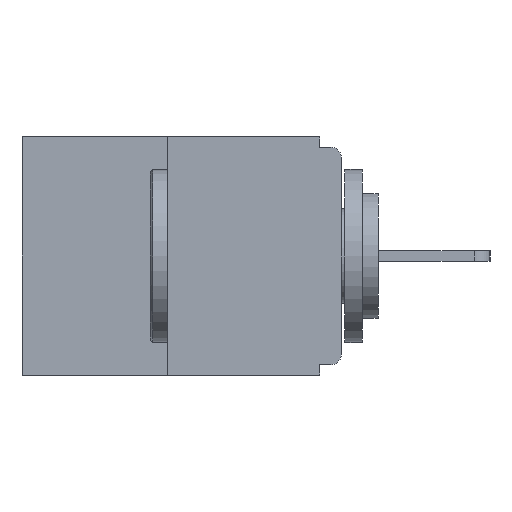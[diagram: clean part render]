
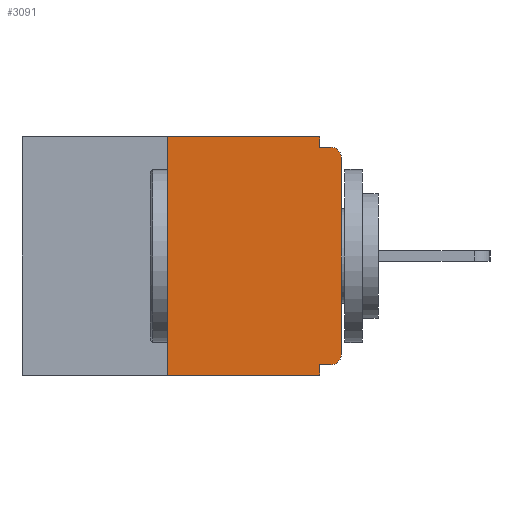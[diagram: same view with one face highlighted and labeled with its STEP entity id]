
A CAD part, left-side view. The second image highlights one B-rep face of the part: STEP entity #3091.
In plain terms, the highlighted planar face has unit normal (-1, 0, 0).
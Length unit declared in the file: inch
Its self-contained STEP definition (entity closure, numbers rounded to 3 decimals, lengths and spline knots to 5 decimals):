
#106 = EDGE_CURVE ( 'NONE', #6109, #9605, #8327, .T. ) ;
#162 = EDGE_CURVE ( 'NONE', #6109, #3119, #6458, .T. ) ;
#165 = EDGE_CURVE ( 'NONE', #1529, #3119, #3879, .T. ) ;
#190 = EDGE_CURVE ( 'NONE', #12623, #11741, #5471, .T. ) ;
#528 = CARTESIAN_POINT ( 'NONE',  ( 0., 0.015, -0.03 ) ) ;
#789 = EDGE_LOOP ( 'NONE', ( #4672, #4776, #4909, #4912, #4935, #4993, #5060, #5098, #5124, #5226 ) ) ;
#1015 = CARTESIAN_POINT ( 'NONE',  ( 0., 0.031, 0. ) ) ;
#1192 = CARTESIAN_POINT ( 'NONE',  ( 0., 0.46, 0. ) ) ;
#1377 = DIRECTION ( 'NONE',  ( 0., 0., 1. ) ) ;
#1440 = DIRECTION ( 'NONE',  ( 0., 1., 0. ) ) ;
#1529 = VERTEX_POINT ( 'NONE', #3378 ) ;
#1629 = VERTEX_POINT ( 'NONE', #12802 ) ;
#1872 = DIRECTION ( 'NONE',  ( 0., 0., -1. ) ) ;
#2788 = CARTESIAN_POINT ( 'NONE',  ( 0., 0.25, 0. ) ) ;
#2852 = LINE ( 'NONE', #1192, #8213 ) ;
#3022 = VERTEX_POINT ( 'NONE', #9345 ) ;
#3091 = ADVANCED_FACE ( 'NONE', ( #6620 ), #8493, .F. ) ;
#3107 = CARTESIAN_POINT ( 'NONE',  ( 0., 0.015, -0.328 ) ) ;
#3119 = VERTEX_POINT ( 'NONE', #13048 ) ;
#3264 = CARTESIAN_POINT ( 'NONE',  ( 0., 0., -0.015 ) ) ;
#3326 = CARTESIAN_POINT ( 'NONE',  ( 0., 0.031, 0. ) ) ;
#3341 = CARTESIAN_POINT ( 'NONE',  ( 0., 0.25, 0. ) ) ;
#3378 = CARTESIAN_POINT ( 'NONE',  ( 0., 0.031, -0.328 ) ) ;
#3797 = CARTESIAN_POINT ( 'NONE',  ( 0., 0.015, -0.313 ) ) ;
#3879 = LINE ( 'NONE', #6142, #11432 ) ;
#4030 = AXIS2_PLACEMENT_3D ( 'NONE', #8640, #5219, #6201 ) ;
#4672 = ORIENTED_EDGE ( 'NONE', *, *, #8890, .F. ) ;
#4776 = ORIENTED_EDGE ( 'NONE', *, *, #106, .F. ) ;
#4909 = ORIENTED_EDGE ( 'NONE', *, *, #162, .T. ) ;
#4912 = ORIENTED_EDGE ( 'NONE', *, *, #165, .F. ) ;
#4935 = ORIENTED_EDGE ( 'NONE', *, *, #6349, .F. ) ;
#4943 = DIRECTION ( 'NONE',  ( 0., 0., -1. ) ) ;
#4993 = ORIENTED_EDGE ( 'NONE', *, *, #7695, .T. ) ;
#5060 = ORIENTED_EDGE ( 'NONE', *, *, #6079, .T. ) ;
#5098 = ORIENTED_EDGE ( 'NONE', *, *, #8484, .T. ) ;
#5124 = ORIENTED_EDGE ( 'NONE', *, *, #7417, .F. ) ;
#5219 = DIRECTION ( 'NONE',  ( 1., 0., 0. ) ) ;
#5226 = ORIENTED_EDGE ( 'NONE', *, *, #190, .F. ) ;
#5432 = CARTESIAN_POINT ( 'NONE',  ( 0., 0.46, -0.343 ) ) ;
#5471 = LINE ( 'NONE', #3326, #13027 ) ;
#5819 = VERTEX_POINT ( 'NONE', #3107 ) ;
#5946 = LINE ( 'NONE', #9600, #10651 ) ;
#5986 = VECTOR ( 'NONE', #1377, 39.37008 ) ;
#6079 = EDGE_CURVE ( 'NONE', #6556, #3022, #5946, .T. ) ;
#6109 = VERTEX_POINT ( 'NONE', #9650 ) ;
#6142 = CARTESIAN_POINT ( 'NONE',  ( 0., 0.031, -0.343 ) ) ;
#6144 = DIRECTION ( 'NONE',  ( 0., 0., -1. ) ) ;
#6201 = DIRECTION ( 'NONE',  ( 0., 0., -1. ) ) ;
#6349 = EDGE_CURVE ( 'NONE', #5819, #1529, #7826, .T. ) ;
#6458 = LINE ( 'NONE', #5432, #9108 ) ;
#6556 = VERTEX_POINT ( 'NONE', #7315 ) ;
#6620 = FACE_OUTER_BOUND ( 'NONE', #789, .T. ) ;
#6659 = DIRECTION ( 'NONE',  ( 0., 0., 1. ) ) ;
#7137 = DIRECTION ( 'NONE',  ( 0., 0., -1. ) ) ;
#7315 = CARTESIAN_POINT ( 'NONE',  ( 0., 0., -0.313 ) ) ;
#7417 = EDGE_CURVE ( 'NONE', #11741, #1629, #11213, .T. ) ;
#7695 = EDGE_CURVE ( 'NONE', #5819, #6556, #7800, .T. ) ;
#7800 = CIRCLE ( 'NONE', #13311, 0.015 ) ;
#7826 = LINE ( 'NONE', #8999, #8132 ) ;
#8132 = VECTOR ( 'NONE', #1440, 39.37008 ) ;
#8213 = VECTOR ( 'NONE', #11827, 39.37008 ) ;
#8219 = AXIS2_PLACEMENT_3D ( 'NONE', #528, #8337, #1872 ) ;
#8327 = LINE ( 'NONE', #2788, #5986 ) ;
#8337 = DIRECTION ( 'NONE',  ( -1., 0., 0. ) ) ;
#8484 = EDGE_CURVE ( 'NONE', #3022, #1629, #12208, .T. ) ;
#8493 = PLANE ( 'NONE',  #4030 ) ;
#8640 = CARTESIAN_POINT ( 'NONE',  ( 0., 0.46, 0. ) ) ;
#8890 = EDGE_CURVE ( 'NONE', #9605, #12623, #2852, .T. ) ;
#8999 = CARTESIAN_POINT ( 'NONE',  ( 0., 0., -0.328 ) ) ;
#9108 = VECTOR ( 'NONE', #10791, 39.37008 ) ;
#9345 = CARTESIAN_POINT ( 'NONE',  ( 0., 0., -0.03 ) ) ;
#9600 = CARTESIAN_POINT ( 'NONE',  ( 0., 0., 0. ) ) ;
#9605 = VERTEX_POINT ( 'NONE', #3341 ) ;
#9650 = CARTESIAN_POINT ( 'NONE',  ( 0., 0.25, -0.343 ) ) ;
#10651 = VECTOR ( 'NONE', #6659, 39.37008 ) ;
#10791 = DIRECTION ( 'NONE',  ( 0., -1., 0. ) ) ;
#10904 = VECTOR ( 'NONE', #13387, 39.37008 ) ;
#10924 = CARTESIAN_POINT ( 'NONE',  ( 0., 0.031, -0.015 ) ) ;
#11011 = DIRECTION ( 'NONE',  ( -1., 0., 0. ) ) ;
#11213 = LINE ( 'NONE', #3264, #10904 ) ;
#11432 = VECTOR ( 'NONE', #7137, 39.37008 ) ;
#11741 = VERTEX_POINT ( 'NONE', #10924 ) ;
#11827 = DIRECTION ( 'NONE',  ( 0., -1., 0. ) ) ;
#12208 = CIRCLE ( 'NONE', #8219, 0.015 ) ;
#12623 = VERTEX_POINT ( 'NONE', #1015 ) ;
#12802 = CARTESIAN_POINT ( 'NONE',  ( 0., 0.015, -0.015 ) ) ;
#13027 = VECTOR ( 'NONE', #6144, 39.37008 ) ;
#13048 = CARTESIAN_POINT ( 'NONE',  ( 0., 0.031, -0.343 ) ) ;
#13311 = AXIS2_PLACEMENT_3D ( 'NONE', #3797, #11011, #4943 ) ;
#13387 = DIRECTION ( 'NONE',  ( 0., -1., 0. ) ) ;
